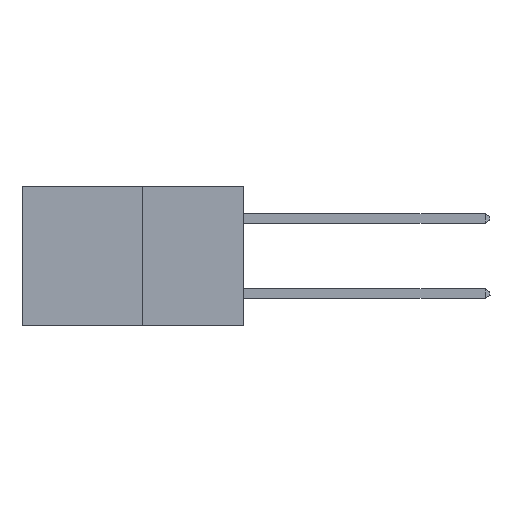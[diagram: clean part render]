
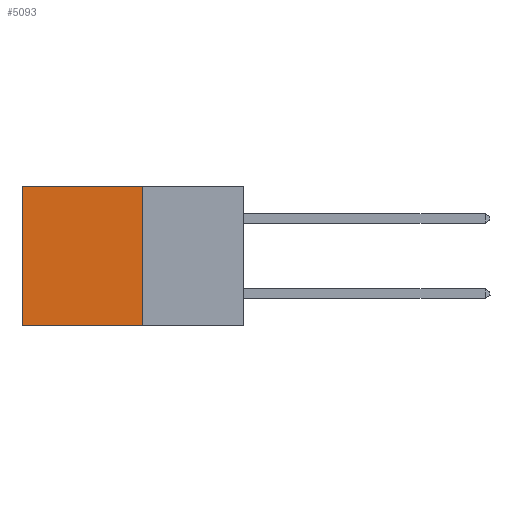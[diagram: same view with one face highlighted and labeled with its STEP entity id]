
A CAD part, left-side view. The second image highlights one B-rep face of the part: STEP entity #5093.
In plain terms, the highlighted planar face has unit normal (-1, 0, 0).
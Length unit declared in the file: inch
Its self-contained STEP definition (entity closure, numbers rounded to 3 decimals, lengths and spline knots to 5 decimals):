
#384 = VECTOR ( 'NONE', #7257, 39.37008 ) ;
#419 = VERTEX_POINT ( 'NONE', #8078 ) ;
#810 = EDGE_CURVE ( 'NONE', #2101, #5779, #2914, .T. ) ;
#1381 = AXIS2_PLACEMENT_3D ( 'NONE', #6602, #4145, #7736 ) ;
#1853 = VERTEX_POINT ( 'NONE', #4305 ) ;
#1953 = ORIENTED_EDGE ( 'NONE', *, *, #810, .F. ) ;
#2034 = ORIENTED_EDGE ( 'NONE', *, *, #5766, .F. ) ;
#2101 = VERTEX_POINT ( 'NONE', #6096 ) ;
#2114 = EDGE_CURVE ( 'NONE', #2101, #1853, #9701, .T. ) ;
#2639 = EDGE_CURVE ( 'NONE', #1853, #419, #3605, .T. ) ;
#2658 = ORIENTED_EDGE ( 'NONE', *, *, #2639, .T. ) ;
#2697 = DIRECTION ( 'NONE',  ( 0., 1., 0. ) ) ;
#2914 = LINE ( 'NONE', #7945, #384 ) ;
#3290 = CARTESIAN_POINT ( 'NONE',  ( 0.277, 0.27, -0.37 ) ) ;
#3314 = DIRECTION ( 'NONE',  ( 0., 0., -1. ) ) ;
#3605 = LINE ( 'NONE', #6333, #9016 ) ;
#3657 = VECTOR ( 'NONE', #8244, 39.37008 ) ;
#3995 = VECTOR ( 'NONE', #2697, 39.37008 ) ;
#4145 = DIRECTION ( 'NONE',  ( 1., 0., 0. ) ) ;
#4305 = CARTESIAN_POINT ( 'NONE',  ( 0.277, 0.59, 0. ) ) ;
#4509 = CARTESIAN_POINT ( 'NONE',  ( 0.277, 0.27, 0. ) ) ;
#4677 = PLANE ( 'NONE',  #1381 ) ;
#5080 = EDGE_LOOP ( 'NONE', ( #2658, #2034, #1953, #9259 ) ) ;
#5093 = ADVANCED_FACE ( 'NONE', ( #7053 ), #4677, .F. ) ;
#5766 = EDGE_CURVE ( 'NONE', #5779, #419, #7905, .T. ) ;
#5779 = VERTEX_POINT ( 'NONE', #3290 ) ;
#6096 = CARTESIAN_POINT ( 'NONE',  ( 0.277, 0.27, 0. ) ) ;
#6333 = CARTESIAN_POINT ( 'NONE',  ( 0.277, 0.59, -0.37 ) ) ;
#6602 = CARTESIAN_POINT ( 'NONE',  ( 0.277, 0.27, -0.37 ) ) ;
#7053 = FACE_OUTER_BOUND ( 'NONE', #5080, .T. ) ;
#7257 = DIRECTION ( 'NONE',  ( 0., 0., -1. ) ) ;
#7736 = DIRECTION ( 'NONE',  ( 0., 0., -1. ) ) ;
#7872 = CARTESIAN_POINT ( 'NONE',  ( 0.277, 0.27, -0.37 ) ) ;
#7905 = LINE ( 'NONE', #7872, #3657 ) ;
#7945 = CARTESIAN_POINT ( 'NONE',  ( 0.277, 0.27, -0.37 ) ) ;
#8078 = CARTESIAN_POINT ( 'NONE',  ( 0.277, 0.59, -0.37 ) ) ;
#8244 = DIRECTION ( 'NONE',  ( 0., 1., 0. ) ) ;
#9016 = VECTOR ( 'NONE', #3314, 39.37008 ) ;
#9259 = ORIENTED_EDGE ( 'NONE', *, *, #2114, .T. ) ;
#9701 = LINE ( 'NONE', #4509, #3995 ) ;
